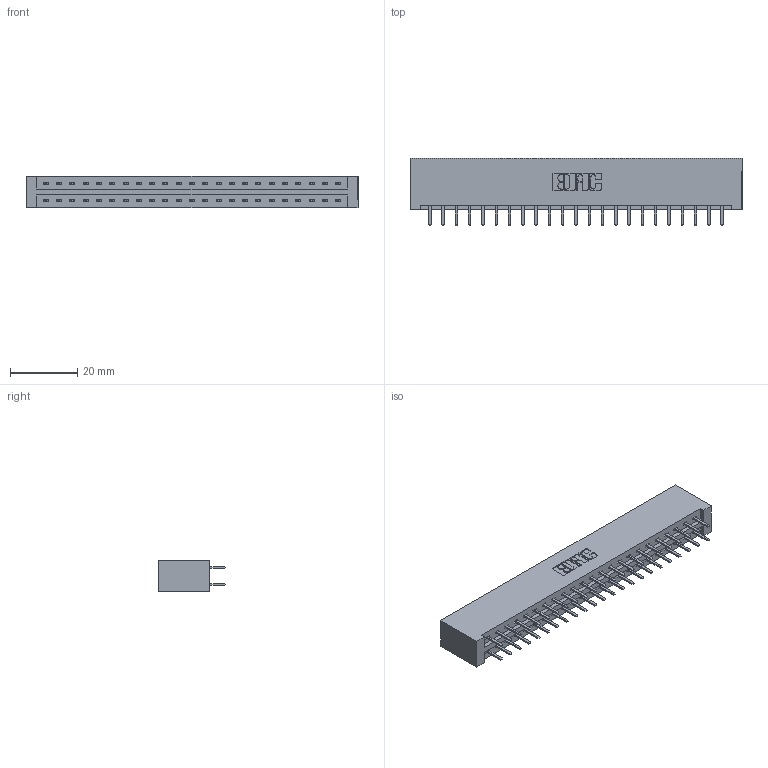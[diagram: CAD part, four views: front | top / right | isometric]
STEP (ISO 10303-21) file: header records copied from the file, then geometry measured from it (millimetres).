
FILE_DESCRIPTION (( 'STEP AP203' ), '1' );
FILE_NAME ('337-046-520-201.STEP', '2019-10-09T13:36:12', ( '' ), ( '' ), 'SwSTEP 2.0', 'SolidWorks 2016', '' );
FILE_SCHEMA (( 'CONFIG_CONTROL_DESIGN' ));
Length unit declared in the file: inch
Products named in the file (3): 345-292-001_345-293-120; 337 Part_No Mounting Lugs; 337-046-520-201
Assembly tree (47 placements, depth 2):
  337-046-520-201
    337 Part_No Mounting Lugs
    345-292-001_345-293-120  x46
Bounding box: 99.01 x 20.02 x 9.4 mm (x, y, z)
Volume: 10922 mm3; surface area: 12161.2 mm2
Topology: 47 solids, 47 shells, 2774 faces, 8061 edges, 5250 vertices
Faces by surface type: plane 1906, cylinder 868
Entity records: 20127 total; most frequent: CARTESIAN_POINT 3418, ORIENTED_EDGE 3342, DIRECTION 2923, EDGE_CURVE 1671, LINE 1547, VECTOR 1547, VERTEX_POINT 1110, AXIS2_PLACEMENT_3D 688
